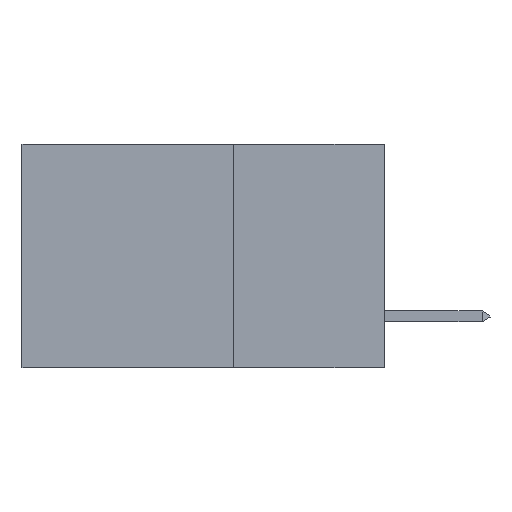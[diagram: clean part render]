
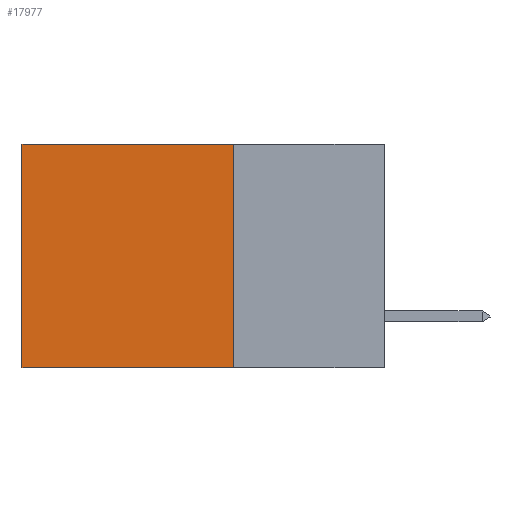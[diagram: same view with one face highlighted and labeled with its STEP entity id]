
A CAD part, left-side view. The second image highlights one B-rep face of the part: STEP entity #17977.
In plain terms, the highlighted planar face has unit normal (-1, 0, 0).
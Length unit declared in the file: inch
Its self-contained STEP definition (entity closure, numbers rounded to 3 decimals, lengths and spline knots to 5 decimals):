
#2075 = CARTESIAN_POINT ( 'NONE',  ( 0.2875, 0.25, 0. ) ) ;
#2241 = VERTEX_POINT ( 'NONE', #8363 ) ;
#3470 = AXIS2_PLACEMENT_3D ( 'NONE', #19627, #21631, #9847 ) ;
#3472 = LINE ( 'NONE', #18779, #13939 ) ;
#5382 = LINE ( 'NONE', #16202, #20415 ) ;
#5541 = CARTESIAN_POINT ( 'NONE',  ( 0.2875, 0.6, -0.37 ) ) ;
#5691 = DIRECTION ( 'NONE',  ( 0., 1., 0. ) ) ;
#5935 = VERTEX_POINT ( 'NONE', #5541 ) ;
#7017 = LINE ( 'NONE', #21861, #16805 ) ;
#7523 = VERTEX_POINT ( 'NONE', #2075 ) ;
#8363 = CARTESIAN_POINT ( 'NONE',  ( 0.2875, 0.25, -0.37 ) ) ;
#9506 = ORIENTED_EDGE ( 'NONE', *, *, #16860, .F. ) ;
#9847 = DIRECTION ( 'NONE',  ( 0., 0., -1. ) ) ;
#11240 = FACE_OUTER_BOUND ( 'NONE', #17100, .T. ) ;
#12529 = EDGE_CURVE ( 'NONE', #19305, #5935, #5382, .T. ) ;
#12853 = DIRECTION ( 'NONE',  ( 0., 1., 0. ) ) ;
#13143 = ORIENTED_EDGE ( 'NONE', *, *, #19329, .F. ) ;
#13939 = VECTOR ( 'NONE', #12853, 39.37008 ) ;
#15170 = LINE ( 'NONE', #23312, #25092 ) ;
#15671 = PLANE ( 'NONE',  #3470 ) ;
#16202 = CARTESIAN_POINT ( 'NONE',  ( 0.2875, 0.6, 0. ) ) ;
#16687 = CARTESIAN_POINT ( 'NONE',  ( 0.2875, 0.6, 0. ) ) ;
#16805 = VECTOR ( 'NONE', #23851, 39.37008 ) ;
#16860 = EDGE_CURVE ( 'NONE', #7523, #2241, #7017, .T. ) ;
#17100 = EDGE_LOOP ( 'NONE', ( #17725, #13143, #9506, #21399 ) ) ;
#17725 = ORIENTED_EDGE ( 'NONE', *, *, #12529, .T. ) ;
#17977 = ADVANCED_FACE ( 'NONE', ( #11240 ), #15671, .F. ) ;
#18200 = DIRECTION ( 'NONE',  ( 0., 0., -1. ) ) ;
#18779 = CARTESIAN_POINT ( 'NONE',  ( 0.2875, 0.25, -0.37 ) ) ;
#18922 = EDGE_CURVE ( 'NONE', #7523, #19305, #15170, .T. ) ;
#19305 = VERTEX_POINT ( 'NONE', #16687 ) ;
#19329 = EDGE_CURVE ( 'NONE', #2241, #5935, #3472, .T. ) ;
#19627 = CARTESIAN_POINT ( 'NONE',  ( 0.2875, 0.25, 0. ) ) ;
#20415 = VECTOR ( 'NONE', #18200, 39.37008 ) ;
#21399 = ORIENTED_EDGE ( 'NONE', *, *, #18922, .T. ) ;
#21631 = DIRECTION ( 'NONE',  ( 1., 0., 0. ) ) ;
#21861 = CARTESIAN_POINT ( 'NONE',  ( 0.2875, 0.25, 0. ) ) ;
#23312 = CARTESIAN_POINT ( 'NONE',  ( 0.2875, 0.25, 0. ) ) ;
#23851 = DIRECTION ( 'NONE',  ( 0., 0., -1. ) ) ;
#25092 = VECTOR ( 'NONE', #5691, 39.37008 ) ;
